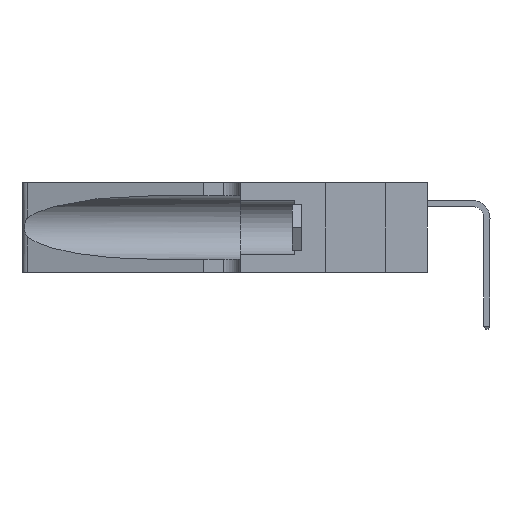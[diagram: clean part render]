
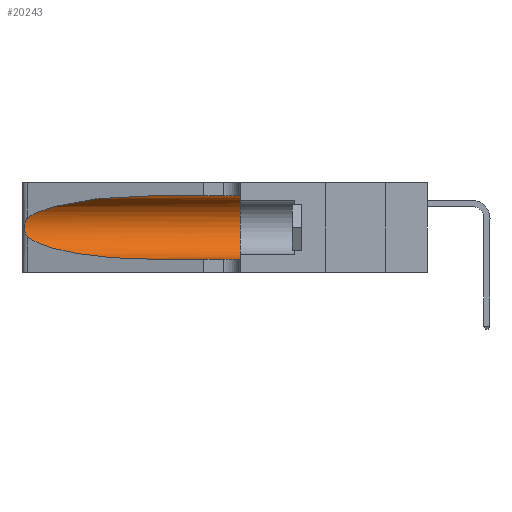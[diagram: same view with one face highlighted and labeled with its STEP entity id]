
A CAD part, left-side view. The second image highlights one B-rep face of the part: STEP entity #20243.
In plain terms, the highlighted cylindrical face has radius 3.308 mm (diameter 6.617 mm), a partial arc.
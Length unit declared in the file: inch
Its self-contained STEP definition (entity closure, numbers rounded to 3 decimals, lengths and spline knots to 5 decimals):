
#1589 = VECTOR ( 'NONE', #28736, 39.37008 ) ;
#2377 = CARTESIAN_POINT ( 'NONE',  ( 0.26075, 1.23896, 0.178 ) ) ;
#3225 = LINE ( 'NONE', #3355, #9397 ) ;
#3355 = CARTESIAN_POINT ( 'NONE',  ( 0.1305, 1.61858, 0.05475 ) ) ;
#4085 = CARTESIAN_POINT ( 'NONE',  ( 0.1305, 0.35, 0.05475 ) ) ;
#4742 = CARTESIAN_POINT ( 'NONE',  ( 0.25856, 1.23593, 0.16098 ) ) ;
#4876 = CARTESIAN_POINT ( 'NONE',  ( 0.1305, 0.72297, 0.05475 ) ) ;
#5203 = ORIENTED_EDGE ( 'NONE', *, *, #16941, .T. ) ;
#5633 = CARTESIAN_POINT ( 'NONE',  ( 0.25487, 1.22718, 0.14631 ) ) ;
#5713 = DIRECTION ( 'NONE',  ( 0., -1., 0. ) ) ;
#6557 = CARTESIAN_POINT ( 'NONE',  ( 0.26018, 1.23835, 0.19895 ) ) ;
#6689 = DIRECTION ( 'NONE',  ( 0., 0., -1. ) ) ;
#6710 = B_SPLINE_CURVE_WITH_KNOTS ( 'NONE', 3,
 ( #20669, #27378, #11562, #27482, #13885, #6557, #16197, #2377, #18462, #4742, #20770, #7058, #23063, #9384 ),
 .UNSPECIFIED., .F., .F.,
 ( 4, 2, 2, 2, 2, 2, 4 ),
 ( 0., 0.00027, 0.00053, 0.00107, 0.0016, 0.00187, 0.00214 ),
 .UNSPECIFIED. ) ;
#7058 = CARTESIAN_POINT ( 'NONE',  ( 0.25639, 1.23186, 0.15144 ) ) ;
#7769 = VERTEX_POINT ( 'NONE', #4085 ) ;
#8481 = LINE ( 'NONE', #12960, #1589 ) ;
#8812 = DIRECTION ( 'NONE',  ( 0., 1., 0. ) ) ;
#9384 = CARTESIAN_POINT ( 'NONE',  ( 0.25487, 1.22718, 0.14631 ) ) ;
#9397 = VECTOR ( 'NONE', #5713, 39.37008 ) ;
#9749 = VERTEX_POINT ( 'NONE', #29097 ) ;
#9915 = FACE_OUTER_BOUND ( 'NONE', #14618, .T. ) ;
#10265 = ORIENTED_EDGE ( 'NONE', *, *, #27288, .F. ) ;
#10370 = ORIENTED_EDGE ( 'NONE', *, *, #20848, .T. ) ;
#11562 = CARTESIAN_POINT ( 'NONE',  ( 0.25639, 1.23184, 0.21858 ) ) ;
#12960 = CARTESIAN_POINT ( 'NONE',  ( 0.1305, 1.61858, 0.31525 ) ) ;
#13487 = CARTESIAN_POINT ( 'NONE',  ( 0.25487, 1.22718, 0.22369 ) ) ;
#13885 = CARTESIAN_POINT ( 'NONE',  ( 0.25854, 1.2359, 0.20912 ) ) ;
#14470 = EDGE_CURVE ( 'NONE', #9749, #21219, #6710, .T. ) ;
#14618 = EDGE_LOOP ( 'NONE', ( #10370, #15502, #5203, #17152, #10265, #20394 ) ) ;
#14993 = CARTESIAN_POINT ( 'NONE',  ( 0.1305, 0.72297, 0.05475 ) ) ;
#15502 = ORIENTED_EDGE ( 'NONE', *, *, #14470, .T. ) ;
#16197 = CARTESIAN_POINT ( 'NONE',  ( 0.26075, 1.23896, 0.19203 ) ) ;
#16227 = CARTESIAN_POINT ( 'NONE',  ( 0.2373, 1.15595, 0.08982 ) ) ;
#16941 = EDGE_CURVE ( 'NONE', #21219, #29572, #22996, .T. ) ;
#17152 = ORIENTED_EDGE ( 'NONE', *, *, #25178, .T. ) ;
#18462 = CARTESIAN_POINT ( 'NONE',  ( 0.26017, 1.23833, 0.17102 ) ) ;
#18584 = CARTESIAN_POINT ( 'NONE',  ( 0.18966, 0.96281, 0.05475 ) ) ;
#18879 = AXIS2_PLACEMENT_3D ( 'NONE', #20309, #20405, #6689 ) ;
#19607 = VERTEX_POINT ( 'NONE', #20246 ) ;
#19690 =( BOUNDED_CURVE ( )  B_SPLINE_CURVE ( 3, ( #20271, #24834, #27079, #13487 ),
 .UNSPECIFIED., .F., .T. ) 
 B_SPLINE_CURVE_WITH_KNOTS ( ( 4, 4 ),
 ( 1.5708, 2.84003 ),
 .UNSPECIFIED. ) 
 CURVE ( )  GEOMETRIC_REPRESENTATION_ITEM ( )  RATIONAL_B_SPLINE_CURVE ( ( 1., 0.87, 0.87, 1. ) ) 
 REPRESENTATION_ITEM ( '' )  );
#20243 = ADVANCED_FACE ( 'NONE', ( #9915 ), #26632, .F. ) ;
#20246 = CARTESIAN_POINT ( 'NONE',  ( 0.1305, 0.35, 0.31525 ) ) ;
#20271 = CARTESIAN_POINT ( 'NONE',  ( 0.1305, 0.72297, 0.31525 ) ) ;
#20309 = CARTESIAN_POINT ( 'NONE',  ( 0.1305, 1.61858, 0.185 ) ) ;
#20394 = ORIENTED_EDGE ( 'NONE', *, *, #27752, .F. ) ;
#20405 = DIRECTION ( 'NONE',  ( 0., -1., 0. ) ) ;
#20669 = CARTESIAN_POINT ( 'NONE',  ( 0.25487, 1.22718, 0.22369 ) ) ;
#20770 = CARTESIAN_POINT ( 'NONE',  ( 0.25789, 1.23486, 0.15765 ) ) ;
#20848 = EDGE_CURVE ( 'NONE', #22679, #9749, #19690, .T. ) ;
#21219 = VERTEX_POINT ( 'NONE', #5633 ) ;
#22112 = CIRCLE ( 'NONE', #24162, 0.13025 ) ;
#22502 = CARTESIAN_POINT ( 'NONE',  ( 0.1305, 0.35, 0.185 ) ) ;
#22679 = VERTEX_POINT ( 'NONE', #28078 ) ;
#22996 =( BOUNDED_CURVE ( )  B_SPLINE_CURVE ( 3, ( #27603, #16227, #18584, #4876 ),
 .UNSPECIFIED., .F., .T. ) 
 B_SPLINE_CURVE_WITH_KNOTS ( ( 4, 4 ),
 ( 3.44316, 4.71239 ),
 .UNSPECIFIED. ) 
 CURVE ( )  GEOMETRIC_REPRESENTATION_ITEM ( )  RATIONAL_B_SPLINE_CURVE ( ( 1., 0.87, 0.87, 1. ) ) 
 REPRESENTATION_ITEM ( '' )  );
#23063 = CARTESIAN_POINT ( 'NONE',  ( 0.25555, 1.22993, 0.14849 ) ) ;
#24162 = AXIS2_PLACEMENT_3D ( 'NONE', #22502, #8812, #24774 ) ;
#24774 = DIRECTION ( 'NONE',  ( 0., 0., 1. ) ) ;
#24834 = CARTESIAN_POINT ( 'NONE',  ( 0.18966, 0.96281, 0.31525 ) ) ;
#25178 = EDGE_CURVE ( 'NONE', #29572, #7769, #3225, .T. ) ;
#26632 = CYLINDRICAL_SURFACE ( 'NONE', #18879, 0.13025 ) ;
#27079 = CARTESIAN_POINT ( 'NONE',  ( 0.2373, 1.15595, 0.28018 ) ) ;
#27288 = EDGE_CURVE ( 'NONE', #19607, #7769, #22112, .T. ) ;
#27378 = CARTESIAN_POINT ( 'NONE',  ( 0.25555, 1.22994, 0.2215 ) ) ;
#27482 = CARTESIAN_POINT ( 'NONE',  ( 0.25787, 1.23484, 0.2124 ) ) ;
#27603 = CARTESIAN_POINT ( 'NONE',  ( 0.25487, 1.22718, 0.14631 ) ) ;
#27752 = EDGE_CURVE ( 'NONE', #22679, #19607, #8481, .T. ) ;
#28078 = CARTESIAN_POINT ( 'NONE',  ( 0.1305, 0.72297, 0.31525 ) ) ;
#28736 = DIRECTION ( 'NONE',  ( 0., -1., 0. ) ) ;
#29097 = CARTESIAN_POINT ( 'NONE',  ( 0.25487, 1.22718, 0.22369 ) ) ;
#29572 = VERTEX_POINT ( 'NONE', #14993 ) ;
